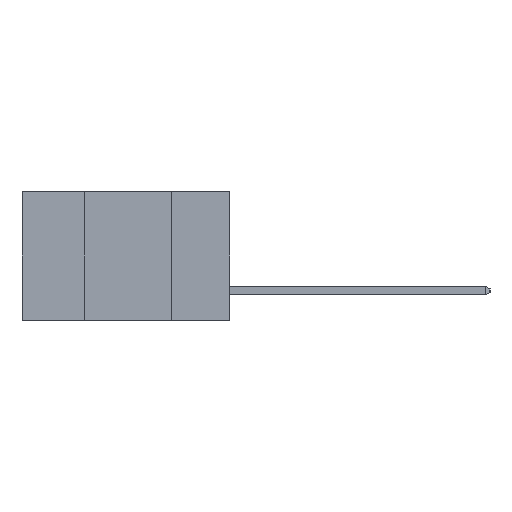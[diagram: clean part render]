
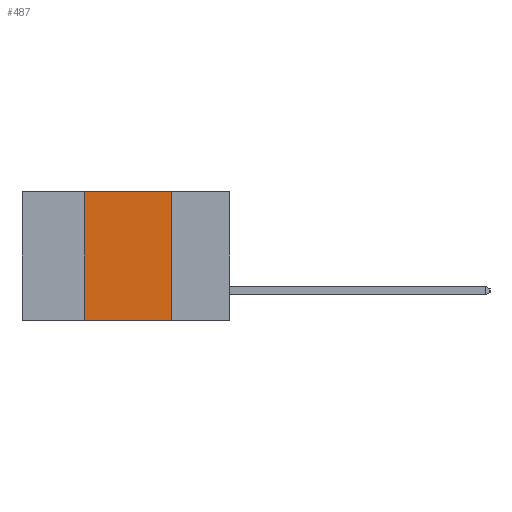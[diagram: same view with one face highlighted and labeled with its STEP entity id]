
A CAD part, left-side view. The second image highlights one B-rep face of the part: STEP entity #487.
In plain terms, the highlighted planar face has unit normal (-1, 0, 0).
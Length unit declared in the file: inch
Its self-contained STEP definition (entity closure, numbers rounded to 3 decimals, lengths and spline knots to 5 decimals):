
#393 = PLANE ( 'NONE',  #1493 ) ;
#475 = VECTOR ( 'NONE', #2456, 39.37008 ) ;
#487 = ADVANCED_FACE ( 'NONE', ( #16747 ), #393, .F. ) ;
#841 = CARTESIAN_POINT ( 'NONE',  ( 0., 0.42, 0. ) ) ;
#984 = DIRECTION ( 'NONE',  ( 0., -1., 0. ) ) ;
#1493 = AXIS2_PLACEMENT_3D ( 'NONE', #15796, #11806, #13162 ) ;
#2456 = DIRECTION ( 'NONE',  ( 0., -1., 0. ) ) ;
#2466 = VERTEX_POINT ( 'NONE', #841 ) ;
#2690 = ORIENTED_EDGE ( 'NONE', *, *, #3128, .F. ) ;
#3128 = EDGE_CURVE ( 'NONE', #2466, #3222, #11178, .T. ) ;
#3222 = VERTEX_POINT ( 'NONE', #16854 ) ;
#3739 = EDGE_CURVE ( 'NONE', #4534, #16484, #4750, .T. ) ;
#3994 = DIRECTION ( 'NONE',  ( 0., 0., 1. ) ) ;
#4056 = CARTESIAN_POINT ( 'NONE',  ( 0., 0.42, -0.37 ) ) ;
#4534 = VERTEX_POINT ( 'NONE', #15046 ) ;
#4750 = LINE ( 'NONE', #9089, #11756 ) ;
#5180 = CARTESIAN_POINT ( 'NONE',  ( 0., 0.6, 0. ) ) ;
#5661 = VECTOR ( 'NONE', #3994, 39.37008 ) ;
#5878 = ORIENTED_EDGE ( 'NONE', *, *, #10916, .F. ) ;
#6302 = ORIENTED_EDGE ( 'NONE', *, *, #16178, .F. ) ;
#7367 = CARTESIAN_POINT ( 'NONE',  ( 0., 0.17, -0.37 ) ) ;
#8617 = CARTESIAN_POINT ( 'NONE',  ( 0., 0.17, -0.37 ) ) ;
#9089 = CARTESIAN_POINT ( 'NONE',  ( 0., 0.6, -0.37 ) ) ;
#9814 = ORIENTED_EDGE ( 'NONE', *, *, #3739, .T. ) ;
#10916 = EDGE_CURVE ( 'NONE', #3222, #16484, #11443, .T. ) ;
#11039 = VECTOR ( 'NONE', #15016, 39.37008 ) ;
#11178 = LINE ( 'NONE', #5180, #475 ) ;
#11443 = LINE ( 'NONE', #7367, #11039 ) ;
#11756 = VECTOR ( 'NONE', #984, 39.37008 ) ;
#11806 = DIRECTION ( 'NONE',  ( 1., 0., 0. ) ) ;
#13162 = DIRECTION ( 'NONE',  ( 0., 0., -1. ) ) ;
#15016 = DIRECTION ( 'NONE',  ( 0., 0., -1. ) ) ;
#15046 = CARTESIAN_POINT ( 'NONE',  ( 0., 0.42, -0.37 ) ) ;
#15503 = LINE ( 'NONE', #4056, #5661 ) ;
#15796 = CARTESIAN_POINT ( 'NONE',  ( 0., 0.6, 0. ) ) ;
#16046 = EDGE_LOOP ( 'NONE', ( #5878, #2690, #6302, #9814 ) ) ;
#16178 = EDGE_CURVE ( 'NONE', #4534, #2466, #15503, .T. ) ;
#16484 = VERTEX_POINT ( 'NONE', #8617 ) ;
#16747 = FACE_OUTER_BOUND ( 'NONE', #16046, .T. ) ;
#16854 = CARTESIAN_POINT ( 'NONE',  ( 0., 0.17, 0. ) ) ;
